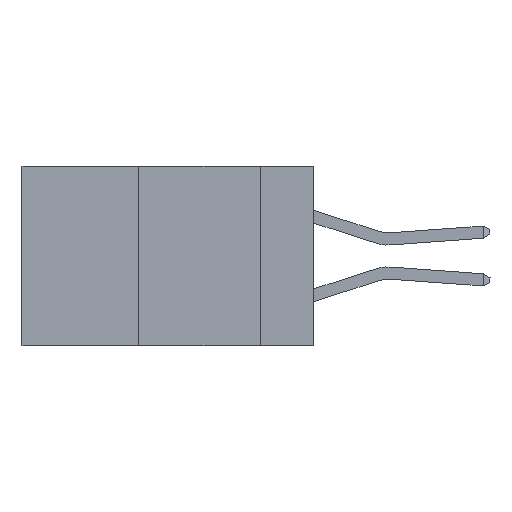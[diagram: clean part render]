
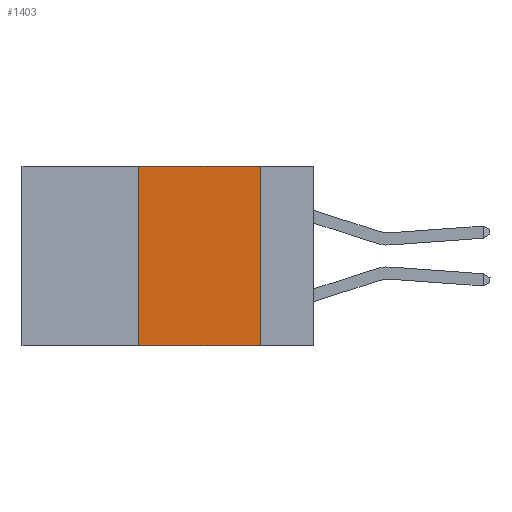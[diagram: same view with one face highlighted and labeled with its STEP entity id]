
A CAD part, left-side view. The second image highlights one B-rep face of the part: STEP entity #1403.
In plain terms, the highlighted planar face has unit normal (-1, 0, 0).
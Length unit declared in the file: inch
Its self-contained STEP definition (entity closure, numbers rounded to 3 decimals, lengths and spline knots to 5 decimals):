
#236 = DIRECTION ( 'NONE',  ( 0., 0., 1. ) ) ;
#314 = ORIENTED_EDGE ( 'NONE', *, *, #9036, .F. ) ;
#1136 = CARTESIAN_POINT ( 'NONE',  ( 0., 0.36, 0. ) ) ;
#1203 = VERTEX_POINT ( 'NONE', #5136 ) ;
#1403 = ADVANCED_FACE ( 'NONE', ( #1442 ), #15747, .F. ) ;
#1442 = FACE_OUTER_BOUND ( 'NONE', #2490, .T. ) ;
#1525 = CARTESIAN_POINT ( 'NONE',  ( 0., 0.11, -0.37 ) ) ;
#1866 = EDGE_CURVE ( 'NONE', #7560, #17663, #18013, .T. ) ;
#2490 = EDGE_LOOP ( 'NONE', ( #314, #16629, #14409, #17830 ) ) ;
#3408 = DIRECTION ( 'NONE',  ( 0., -1., 0. ) ) ;
#4434 = VECTOR ( 'NONE', #15800, 39.37008 ) ;
#5136 = CARTESIAN_POINT ( 'NONE',  ( 0., 0.11, 0. ) ) ;
#5496 = DIRECTION ( 'NONE',  ( 0., -1., 0. ) ) ;
#6037 = EDGE_CURVE ( 'NONE', #17663, #1203, #7613, .T. ) ;
#6100 = DIRECTION ( 'NONE',  ( 1., 0., 0. ) ) ;
#6196 = VERTEX_POINT ( 'NONE', #1525 ) ;
#6360 = VECTOR ( 'NONE', #5496, 39.37008 ) ;
#6501 = VECTOR ( 'NONE', #236, 39.37008 ) ;
#7560 = VERTEX_POINT ( 'NONE', #9795 ) ;
#7613 = LINE ( 'NONE', #19794, #6360 ) ;
#7913 = CARTESIAN_POINT ( 'NONE',  ( 0., 0.11, 0. ) ) ;
#8213 = EDGE_CURVE ( 'NONE', #7560, #6196, #20821, .T. ) ;
#8537 = CARTESIAN_POINT ( 'NONE',  ( 0., 0.36, 0. ) ) ;
#9036 = EDGE_CURVE ( 'NONE', #1203, #6196, #10243, .T. ) ;
#9795 = CARTESIAN_POINT ( 'NONE',  ( 0., 0.36, -0.37 ) ) ;
#10243 = LINE ( 'NONE', #7913, #4434 ) ;
#10290 = VECTOR ( 'NONE', #3408, 39.37008 ) ;
#12735 = DIRECTION ( 'NONE',  ( 0., 0., -1. ) ) ;
#14409 = ORIENTED_EDGE ( 'NONE', *, *, #1866, .F. ) ;
#15747 = PLANE ( 'NONE',  #16165 ) ;
#15800 = DIRECTION ( 'NONE',  ( 0., 0., -1. ) ) ;
#16165 = AXIS2_PLACEMENT_3D ( 'NONE', #20462, #6100, #12735 ) ;
#16629 = ORIENTED_EDGE ( 'NONE', *, *, #6037, .F. ) ;
#17663 = VERTEX_POINT ( 'NONE', #1136 ) ;
#17824 = CARTESIAN_POINT ( 'NONE',  ( 0., 0.6, -0.37 ) ) ;
#17830 = ORIENTED_EDGE ( 'NONE', *, *, #8213, .T. ) ;
#18013 = LINE ( 'NONE', #8537, #6501 ) ;
#19794 = CARTESIAN_POINT ( 'NONE',  ( 0., 0.6, 0. ) ) ;
#20462 = CARTESIAN_POINT ( 'NONE',  ( 0., 0.6, 0. ) ) ;
#20821 = LINE ( 'NONE', #17824, #10290 ) ;
